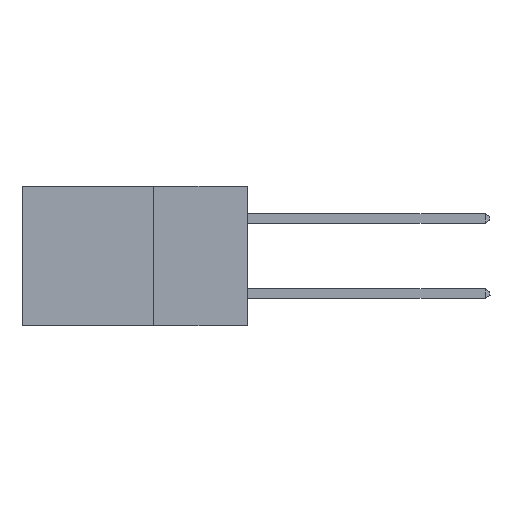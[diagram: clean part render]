
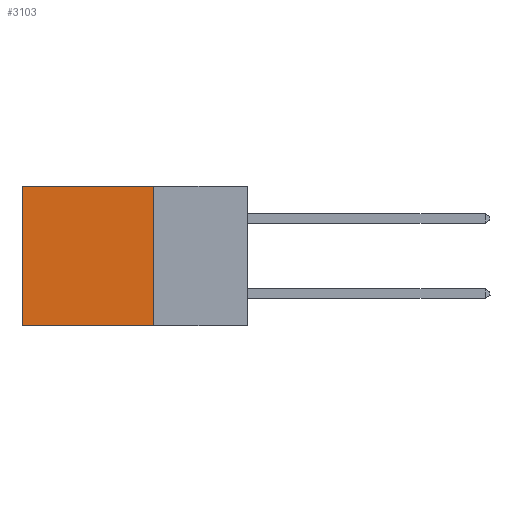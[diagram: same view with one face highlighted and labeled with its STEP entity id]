
A CAD part, left-side view. The second image highlights one B-rep face of the part: STEP entity #3103.
In plain terms, the highlighted planar face has unit normal (-1, 0, 0).
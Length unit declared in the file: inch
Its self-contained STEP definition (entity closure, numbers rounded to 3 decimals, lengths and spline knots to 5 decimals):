
#1049 = VECTOR ( 'NONE', #22701, 39.37008 ) ;
#1625 = VERTEX_POINT ( 'NONE', #16364 ) ;
#2332 = DIRECTION ( 'NONE',  ( 0., 1., 0. ) ) ;
#2765 = CARTESIAN_POINT ( 'NONE',  ( 0.298, 0.6, -0.37 ) ) ;
#2834 = DIRECTION ( 'NONE',  ( 1., 0., 0. ) ) ;
#3006 = CARTESIAN_POINT ( 'NONE',  ( 0.298, 0.25, 0. ) ) ;
#3103 = ADVANCED_FACE ( 'NONE', ( #13263 ), #27591, .F. ) ;
#3336 = AXIS2_PLACEMENT_3D ( 'NONE', #16377, #2834, #18702 ) ;
#3848 = CARTESIAN_POINT ( 'NONE',  ( 0.298, 0.25, -0.37 ) ) ;
#4069 = DIRECTION ( 'NONE',  ( 0., 0., -1. ) ) ;
#4397 = VERTEX_POINT ( 'NONE', #2765 ) ;
#6582 = ORIENTED_EDGE ( 'NONE', *, *, #11449, .F. ) ;
#7395 = VERTEX_POINT ( 'NONE', #28747 ) ;
#8353 = EDGE_CURVE ( 'NONE', #1625, #7395, #11442, .T. ) ;
#8565 = LINE ( 'NONE', #20449, #1049 ) ;
#9124 = CARTESIAN_POINT ( 'NONE',  ( 0.298, 0.25, -0.37 ) ) ;
#9812 = ORIENTED_EDGE ( 'NONE', *, *, #13299, .T. ) ;
#9857 = LINE ( 'NONE', #10901, #27092 ) ;
#10901 = CARTESIAN_POINT ( 'NONE',  ( 0.298, 0.6, 0. ) ) ;
#11442 = LINE ( 'NONE', #3006, #27972 ) ;
#11449 = EDGE_CURVE ( 'NONE', #1625, #18120, #8565, .T. ) ;
#13263 = FACE_OUTER_BOUND ( 'NONE', #24102, .T. ) ;
#13299 = EDGE_CURVE ( 'NONE', #7395, #4397, #9857, .T. ) ;
#16364 = CARTESIAN_POINT ( 'NONE',  ( 0.298, 0.25, 0. ) ) ;
#16377 = CARTESIAN_POINT ( 'NONE',  ( 0.298, 0.25, 0. ) ) ;
#18120 = VERTEX_POINT ( 'NONE', #3848 ) ;
#18702 = DIRECTION ( 'NONE',  ( 0., 0., -1. ) ) ;
#18864 = DIRECTION ( 'NONE',  ( 0., 1., 0. ) ) ;
#20449 = CARTESIAN_POINT ( 'NONE',  ( 0.298, 0.25, 0. ) ) ;
#20823 = LINE ( 'NONE', #9124, #26065 ) ;
#22580 = ORIENTED_EDGE ( 'NONE', *, *, #8353, .T. ) ;
#22701 = DIRECTION ( 'NONE',  ( 0., 0., -1. ) ) ;
#23739 = EDGE_CURVE ( 'NONE', #18120, #4397, #20823, .T. ) ;
#24084 = ORIENTED_EDGE ( 'NONE', *, *, #23739, .F. ) ;
#24102 = EDGE_LOOP ( 'NONE', ( #9812, #24084, #6582, #22580 ) ) ;
#26065 = VECTOR ( 'NONE', #2332, 39.37008 ) ;
#27092 = VECTOR ( 'NONE', #4069, 39.37008 ) ;
#27591 = PLANE ( 'NONE',  #3336 ) ;
#27972 = VECTOR ( 'NONE', #18864, 39.37008 ) ;
#28747 = CARTESIAN_POINT ( 'NONE',  ( 0.298, 0.6, 0. ) ) ;
